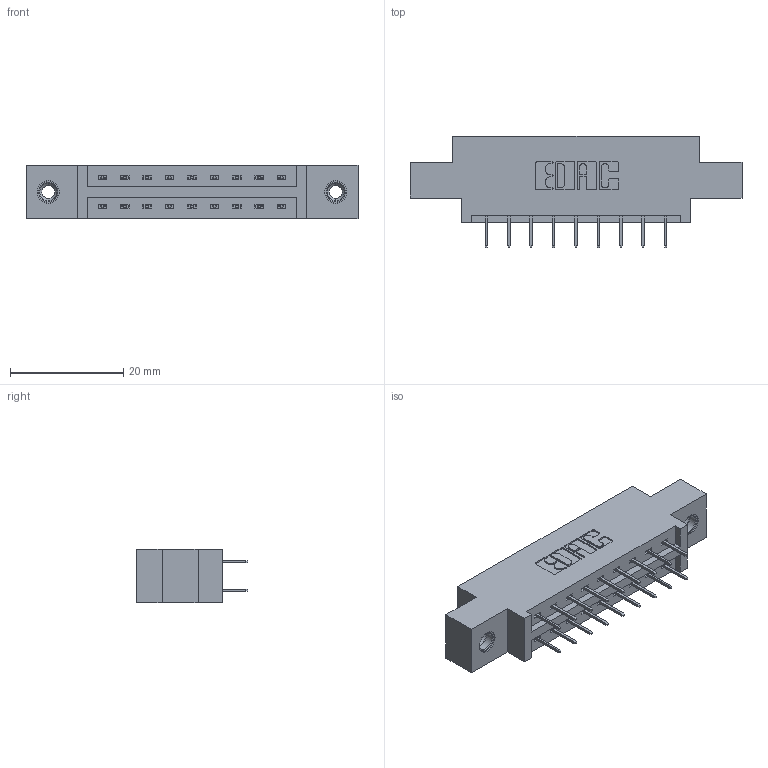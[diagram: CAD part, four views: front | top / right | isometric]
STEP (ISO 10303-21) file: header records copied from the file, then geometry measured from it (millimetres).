
FILE_DESCRIPTION (( 'STEP AP203' ), '1' );
FILE_NAME ('337-018-524-808.STEP', '2018-08-05T00:27:42', ( '' ), ( '' ), 'SwSTEP 2.0', 'SolidWorks 2016', '' );
FILE_SCHEMA (( 'CONFIG_CONTROL_DESIGN' ));
Length unit declared in the file: inch
Products named in the file (4): 337 Part_0.170 Offset - 0.156 Dia-TI; 345-292-001_345-293-124; 345-250-001_345-250-003-102; 337-018-524-808
Assembly tree (21 placements, depth 2):
  337-018-524-808
    337 Part_0.170 Offset - 0.156 Dia-TI
    345-292-001_345-293-124  x18
    345-250-001_345-250-003-102  x2
Bounding box: 58.67 x 19.69 x 9.4 mm (x, y, z)
Volume: 5593 mm3; surface area: 6049.7 mm2
Topology: 21 solids, 21 shells, 1222 faces, 3429 edges, 2206 vertices
Faces by surface type: plane 898, cylinder 308, cone 12, torus 4
Entity records: 12638 total; most frequent: CARTESIAN_POINT 2137, ORIENTED_EDGE 2066, DIRECTION 1911, EDGE_CURVE 1033, LINE 889, VECTOR 889, VERTEX_POINT 680, AXIS2_PLACEMENT_3D 511
